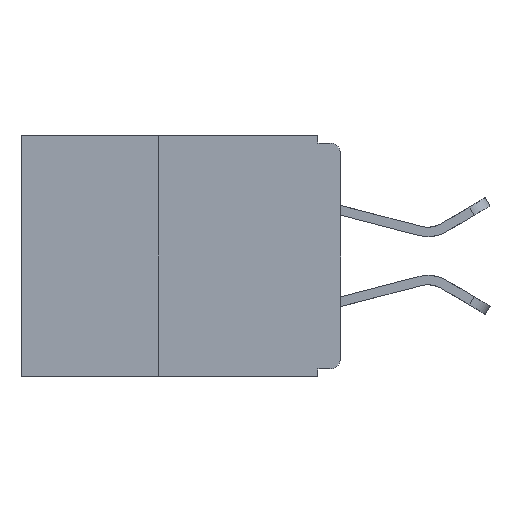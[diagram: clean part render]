
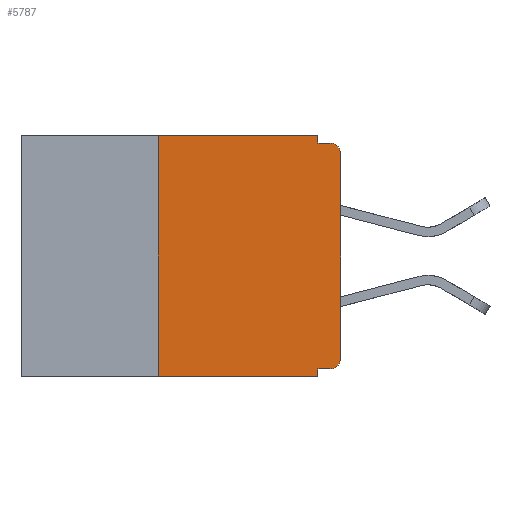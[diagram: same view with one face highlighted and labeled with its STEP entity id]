
A CAD part, left-side view. The second image highlights one B-rep face of the part: STEP entity #5787.
In plain terms, the highlighted planar face has unit normal (-1, 0, 0).
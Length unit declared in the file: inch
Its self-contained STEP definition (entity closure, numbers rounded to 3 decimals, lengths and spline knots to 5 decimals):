
#30 = DIRECTION ( 'NONE',  ( 0., 0., 1. ) ) ;
#62 = VERTEX_POINT ( 'NONE', #11919 ) ;
#232 = VECTOR ( 'NONE', #6642, 39.37008 ) ;
#250 = CARTESIAN_POINT ( 'NONE',  ( 0., 0.031, -0.33 ) ) ;
#388 = CARTESIAN_POINT ( 'NONE',  ( 0., 0.437, -0.33 ) ) ;
#569 = VECTOR ( 'NONE', #7922, 39.37008 ) ;
#616 = ORIENTED_EDGE ( 'NONE', *, *, #3219, .T. ) ;
#619 = AXIS2_PLACEMENT_3D ( 'NONE', #11973, #4672, #12012 ) ;
#662 = CARTESIAN_POINT ( 'NONE',  ( 0., 0.015, -0.32 ) ) ;
#728 = ORIENTED_EDGE ( 'NONE', *, *, #11736, .T. ) ;
#750 = VERTEX_POINT ( 'NONE', #13716 ) ;
#945 = LINE ( 'NONE', #7987, #569 ) ;
#993 = DIRECTION ( 'NONE',  ( 0., -1., 0. ) ) ;
#995 = VECTOR ( 'NONE', #5476, 39.37008 ) ;
#1035 = VERTEX_POINT ( 'NONE', #250 ) ;
#1392 = CARTESIAN_POINT ( 'NONE',  ( 0., 0.437, 0. ) ) ;
#1883 = ORIENTED_EDGE ( 'NONE', *, *, #4056, .F. ) ;
#1891 = ORIENTED_EDGE ( 'NONE', *, *, #4020, .F. ) ;
#1954 = VECTOR ( 'NONE', #8921, 39.37008 ) ;
#1984 = VERTEX_POINT ( 'NONE', #662 ) ;
#2177 = EDGE_CURVE ( 'NONE', #8002, #1035, #6741, .T. ) ;
#2627 = ORIENTED_EDGE ( 'NONE', *, *, #8582, .T. ) ;
#2720 = CARTESIAN_POINT ( 'NONE',  ( 0., 0., -0.025 ) ) ;
#2956 = DIRECTION ( 'NONE',  ( -1., 0., 0. ) ) ;
#3219 = EDGE_CURVE ( 'NONE', #12211, #7157, #7500, .T. ) ;
#3601 = VECTOR ( 'NONE', #5338, 39.37008 ) ;
#3634 = ORIENTED_EDGE ( 'NONE', *, *, #9731, .F. ) ;
#3639 = ORIENTED_EDGE ( 'NONE', *, *, #2177, .F. ) ;
#3644 = CIRCLE ( 'NONE', #9055, 0.015 ) ;
#4020 = EDGE_CURVE ( 'NONE', #1984, #8002, #945, .T. ) ;
#4056 = EDGE_CURVE ( 'NONE', #7935, #8294, #8795, .T. ) ;
#4090 = DIRECTION ( 'NONE',  ( 0., 0., 1. ) ) ;
#4220 = EDGE_CURVE ( 'NONE', #750, #7935, #6840, .T. ) ;
#4334 = CARTESIAN_POINT ( 'NONE',  ( 0., 0., 0. ) ) ;
#4672 = DIRECTION ( 'NONE',  ( 1., 0., 0. ) ) ;
#4689 = VECTOR ( 'NONE', #30, 39.37008 ) ;
#5180 = LINE ( 'NONE', #388, #1954 ) ;
#5338 = DIRECTION ( 'NONE',  ( 0., -1., 0. ) ) ;
#5414 = EDGE_CURVE ( 'NONE', #7157, #6307, #3644, .T. ) ;
#5476 = DIRECTION ( 'NONE',  ( 0., 0., -1. ) ) ;
#5749 = LINE ( 'NONE', #9397, #8169 ) ;
#5787 = ADVANCED_FACE ( 'NONE', ( #12960 ), #8869, .F. ) ;
#6307 = VERTEX_POINT ( 'NONE', #7660 ) ;
#6516 = DIRECTION ( 'NONE',  ( -1., 0., 0. ) ) ;
#6554 = CARTESIAN_POINT ( 'NONE',  ( 0., 0.031, -0.32 ) ) ;
#6642 = DIRECTION ( 'NONE',  ( 0., 0., -1. ) ) ;
#6650 = CARTESIAN_POINT ( 'NONE',  ( 0., 0., -0.305 ) ) ;
#6741 = LINE ( 'NONE', #8619, #995 ) ;
#6765 = EDGE_CURVE ( 'NONE', #8294, #6307, #6785, .T. ) ;
#6785 = LINE ( 'NONE', #9486, #3601 ) ;
#6840 = LINE ( 'NONE', #1392, #12367 ) ;
#6973 = ORIENTED_EDGE ( 'NONE', *, *, #5414, .T. ) ;
#7157 = VERTEX_POINT ( 'NONE', #2720 ) ;
#7297 = CARTESIAN_POINT ( 'NONE',  ( 0., 0.031, 0. ) ) ;
#7500 = LINE ( 'NONE', #4334, #4689 ) ;
#7506 = DIRECTION ( 'NONE',  ( 0., 0., -1. ) ) ;
#7660 = CARTESIAN_POINT ( 'NONE',  ( 0., 0.015, -0.01 ) ) ;
#7922 = DIRECTION ( 'NONE',  ( 0., 1., 0. ) ) ;
#7935 = VERTEX_POINT ( 'NONE', #11463 ) ;
#7987 = CARTESIAN_POINT ( 'NONE',  ( 0., 0., -0.32 ) ) ;
#8002 = VERTEX_POINT ( 'NONE', #6554 ) ;
#8169 = VECTOR ( 'NONE', #4090, 39.37008 ) ;
#8294 = VERTEX_POINT ( 'NONE', #9097 ) ;
#8582 = EDGE_CURVE ( 'NONE', #1984, #12211, #10494, .T. ) ;
#8619 = CARTESIAN_POINT ( 'NONE',  ( 0., 0.031, -0.33 ) ) ;
#8795 = LINE ( 'NONE', #7297, #232 ) ;
#8869 = PLANE ( 'NONE',  #619 ) ;
#8921 = DIRECTION ( 'NONE',  ( 0., -1., 0. ) ) ;
#9055 = AXIS2_PLACEMENT_3D ( 'NONE', #9347, #2956, #10383 ) ;
#9097 = CARTESIAN_POINT ( 'NONE',  ( 0., 0.031, -0.01 ) ) ;
#9347 = CARTESIAN_POINT ( 'NONE',  ( 0., 0.015, -0.025 ) ) ;
#9397 = CARTESIAN_POINT ( 'NONE',  ( 0., 0.25, -0.33 ) ) ;
#9486 = CARTESIAN_POINT ( 'NONE',  ( 0., 0., -0.01 ) ) ;
#9731 = EDGE_CURVE ( 'NONE', #62, #750, #5749, .T. ) ;
#10383 = DIRECTION ( 'NONE',  ( 0., 0., -1. ) ) ;
#10494 = CIRCLE ( 'NONE', #11275, 0.015 ) ;
#11275 = AXIS2_PLACEMENT_3D ( 'NONE', #12702, #6516, #7506 ) ;
#11325 = EDGE_LOOP ( 'NONE', ( #616, #6973, #12453, #1883, #13260, #3634, #728, #3639, #1891, #2627 ) ) ;
#11463 = CARTESIAN_POINT ( 'NONE',  ( 0., 0.031, 0. ) ) ;
#11736 = EDGE_CURVE ( 'NONE', #62, #1035, #5180, .T. ) ;
#11919 = CARTESIAN_POINT ( 'NONE',  ( 0., 0.25, -0.33 ) ) ;
#11973 = CARTESIAN_POINT ( 'NONE',  ( 0., 0.437, 0. ) ) ;
#12012 = DIRECTION ( 'NONE',  ( 0., 0., -1. ) ) ;
#12211 = VERTEX_POINT ( 'NONE', #6650 ) ;
#12367 = VECTOR ( 'NONE', #993, 39.37008 ) ;
#12453 = ORIENTED_EDGE ( 'NONE', *, *, #6765, .F. ) ;
#12702 = CARTESIAN_POINT ( 'NONE',  ( 0., 0.015, -0.305 ) ) ;
#12960 = FACE_OUTER_BOUND ( 'NONE', #11325, .T. ) ;
#13260 = ORIENTED_EDGE ( 'NONE', *, *, #4220, .F. ) ;
#13716 = CARTESIAN_POINT ( 'NONE',  ( 0., 0.25, 0. ) ) ;
